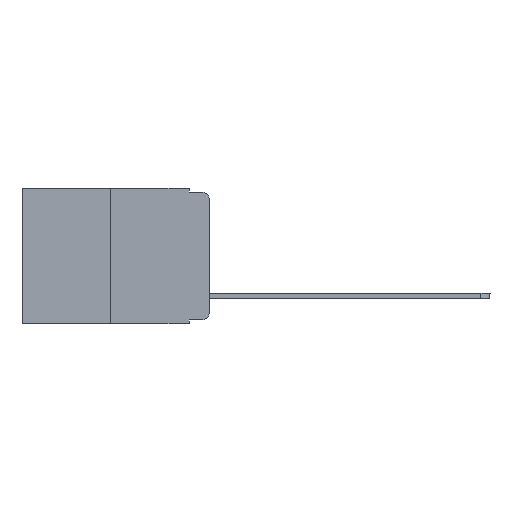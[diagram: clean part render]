
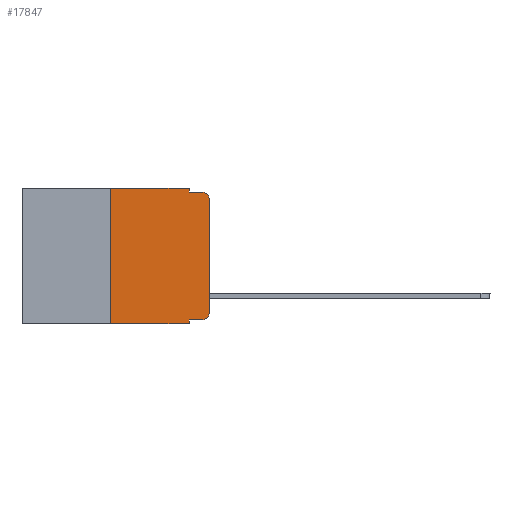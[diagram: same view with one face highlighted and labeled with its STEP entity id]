
A CAD part, left-side view. The second image highlights one B-rep face of the part: STEP entity #17847.
In plain terms, the highlighted planar face has unit normal (-1, 0, 0).
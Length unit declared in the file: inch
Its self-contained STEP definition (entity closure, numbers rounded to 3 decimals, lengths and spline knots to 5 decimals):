
#158 = CARTESIAN_POINT ( 'NONE',  ( 0., 0.25, -0.343 ) ) ;
#547 = VERTEX_POINT ( 'NONE', #12918 ) ;
#594 = ORIENTED_EDGE ( 'NONE', *, *, #1044, .F. ) ;
#619 = ORIENTED_EDGE ( 'NONE', *, *, #7088, .F. ) ;
#668 = ORIENTED_EDGE ( 'NONE', *, *, #2728, .F. ) ;
#829 = VERTEX_POINT ( 'NONE', #16306 ) ;
#845 = VERTEX_POINT ( 'NONE', #3583 ) ;
#1044 = EDGE_CURVE ( 'NONE', #845, #12829, #3984, .T. ) ;
#1314 = CARTESIAN_POINT ( 'NONE',  ( 0., 0.02, -0.01 ) ) ;
#1320 = EDGE_CURVE ( 'NONE', #5961, #4946, #11878, .T. ) ;
#1336 = CARTESIAN_POINT ( 'NONE',  ( 0., 0.473, 0. ) ) ;
#1972 = AXIS2_PLACEMENT_3D ( 'NONE', #3165, #6130, #17148 ) ;
#2025 = EDGE_CURVE ( 'NONE', #11374, #6385, #9630, .T. ) ;
#2032 = CARTESIAN_POINT ( 'NONE',  ( 0., 0.051, -0.333 ) ) ;
#2348 = AXIS2_PLACEMENT_3D ( 'NONE', #1336, #13784, #17980 ) ;
#2728 = EDGE_CURVE ( 'NONE', #5961, #17198, #5700, .T. ) ;
#2887 = DIRECTION ( 'NONE',  ( 0., 0., 1. ) ) ;
#3105 = EDGE_LOOP ( 'NONE', ( #15650, #14796, #594, #16185, #15342, #619, #8765, #668, #8540, #15934 ) ) ;
#3165 = CARTESIAN_POINT ( 'NONE',  ( 0., 0.02, -0.03 ) ) ;
#3209 = VECTOR ( 'NONE', #2887, 39.37008 ) ;
#3583 = CARTESIAN_POINT ( 'NONE',  ( 0., 0.051, -0.01 ) ) ;
#3816 = VERTEX_POINT ( 'NONE', #158 ) ;
#3984 = LINE ( 'NONE', #5981, #8115 ) ;
#4218 = CARTESIAN_POINT ( 'NONE',  ( 0., 0., 0. ) ) ;
#4498 = CARTESIAN_POINT ( 'NONE',  ( 0., 0.25, 0. ) ) ;
#4946 = VERTEX_POINT ( 'NONE', #5100 ) ;
#5100 = CARTESIAN_POINT ( 'NONE',  ( 0., 0.02, -0.333 ) ) ;
#5335 = FACE_OUTER_BOUND ( 'NONE', #3105, .T. ) ;
#5687 = DIRECTION ( 'NONE',  ( 0., -1., 0. ) ) ;
#5700 = LINE ( 'NONE', #17132, #13160 ) ;
#5760 = CARTESIAN_POINT ( 'NONE',  ( 0., 0.051, 0. ) ) ;
#5932 = CARTESIAN_POINT ( 'NONE',  ( 0., 0.051, -0.333 ) ) ;
#5961 = VERTEX_POINT ( 'NONE', #2032 ) ;
#5981 = CARTESIAN_POINT ( 'NONE',  ( 0., 0.051, -0.01 ) ) ;
#6130 = DIRECTION ( 'NONE',  ( -1., 0., 0. ) ) ;
#6385 = VERTEX_POINT ( 'NONE', #12574 ) ;
#6959 = AXIS2_PLACEMENT_3D ( 'NONE', #15622, #14139, #17008 ) ;
#7088 = EDGE_CURVE ( 'NONE', #3816, #11374, #7486, .T. ) ;
#7486 = LINE ( 'NONE', #4498, #17756 ) ;
#7660 = DIRECTION ( 'NONE',  ( 0., -1., 0. ) ) ;
#7775 = LINE ( 'NONE', #4218, #3209 ) ;
#7902 = VECTOR ( 'NONE', #13980, 39.37008 ) ;
#8012 = LINE ( 'NONE', #11239, #15036 ) ;
#8024 = VECTOR ( 'NONE', #15513, 39.37008 ) ;
#8115 = VECTOR ( 'NONE', #7660, 39.37008 ) ;
#8540 = ORIENTED_EDGE ( 'NONE', *, *, #1320, .T. ) ;
#8765 = ORIENTED_EDGE ( 'NONE', *, *, #16663, .T. ) ;
#9630 = LINE ( 'NONE', #9839, #7902 ) ;
#9839 = CARTESIAN_POINT ( 'NONE',  ( 0., 0.473, 0. ) ) ;
#9876 = VECTOR ( 'NONE', #11562, 39.37008 ) ;
#9952 = CIRCLE ( 'NONE', #6959, 0.02 ) ;
#10377 = DIRECTION ( 'NONE',  ( 0., 0., -1. ) ) ;
#11239 = CARTESIAN_POINT ( 'NONE',  ( 0., 0.473, -0.343 ) ) ;
#11374 = VERTEX_POINT ( 'NONE', #11830 ) ;
#11390 = DIRECTION ( 'NONE',  ( 0., 0., 1. ) ) ;
#11562 = DIRECTION ( 'NONE',  ( 0., -1., 0. ) ) ;
#11819 = EDGE_CURVE ( 'NONE', #6385, #845, #13310, .T. ) ;
#11830 = CARTESIAN_POINT ( 'NONE',  ( 0., 0.25, 0. ) ) ;
#11878 = LINE ( 'NONE', #5932, #9876 ) ;
#12436 = PLANE ( 'NONE',  #2348 ) ;
#12574 = CARTESIAN_POINT ( 'NONE',  ( 0., 0.051, 0. ) ) ;
#12829 = VERTEX_POINT ( 'NONE', #1314 ) ;
#12918 = CARTESIAN_POINT ( 'NONE',  ( 0., 0., -0.313 ) ) ;
#13160 = VECTOR ( 'NONE', #10377, 39.37008 ) ;
#13310 = LINE ( 'NONE', #5760, #8024 ) ;
#13784 = DIRECTION ( 'NONE',  ( 1., 0., 0. ) ) ;
#13980 = DIRECTION ( 'NONE',  ( 0., -1., 0. ) ) ;
#14139 = DIRECTION ( 'NONE',  ( -1., 0., 0. ) ) ;
#14796 = ORIENTED_EDGE ( 'NONE', *, *, #16177, .T. ) ;
#15036 = VECTOR ( 'NONE', #5687, 39.37008 ) ;
#15342 = ORIENTED_EDGE ( 'NONE', *, *, #2025, .F. ) ;
#15475 = CARTESIAN_POINT ( 'NONE',  ( 0., 0.051, -0.343 ) ) ;
#15513 = DIRECTION ( 'NONE',  ( 0., 0., -1. ) ) ;
#15622 = CARTESIAN_POINT ( 'NONE',  ( 0., 0.02, -0.313 ) ) ;
#15650 = ORIENTED_EDGE ( 'NONE', *, *, #17331, .T. ) ;
#15934 = ORIENTED_EDGE ( 'NONE', *, *, #16688, .T. ) ;
#16177 = EDGE_CURVE ( 'NONE', #829, #12829, #16800, .T. ) ;
#16185 = ORIENTED_EDGE ( 'NONE', *, *, #11819, .F. ) ;
#16306 = CARTESIAN_POINT ( 'NONE',  ( 0., 0., -0.03 ) ) ;
#16663 = EDGE_CURVE ( 'NONE', #3816, #17198, #8012, .T. ) ;
#16688 = EDGE_CURVE ( 'NONE', #4946, #547, #9952, .T. ) ;
#16800 = CIRCLE ( 'NONE', #1972, 0.02 ) ;
#17008 = DIRECTION ( 'NONE',  ( 0., 0., -1. ) ) ;
#17132 = CARTESIAN_POINT ( 'NONE',  ( 0., 0.051, 0. ) ) ;
#17148 = DIRECTION ( 'NONE',  ( 0., 0., -1. ) ) ;
#17198 = VERTEX_POINT ( 'NONE', #15475 ) ;
#17331 = EDGE_CURVE ( 'NONE', #547, #829, #7775, .T. ) ;
#17756 = VECTOR ( 'NONE', #11390, 39.37008 ) ;
#17847 = ADVANCED_FACE ( 'NONE', ( #5335 ), #12436, .F. ) ;
#17980 = DIRECTION ( 'NONE',  ( 0., 0., -1. ) ) ;
